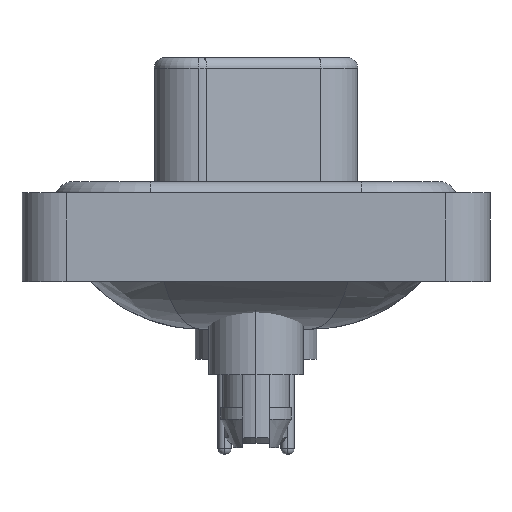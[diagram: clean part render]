
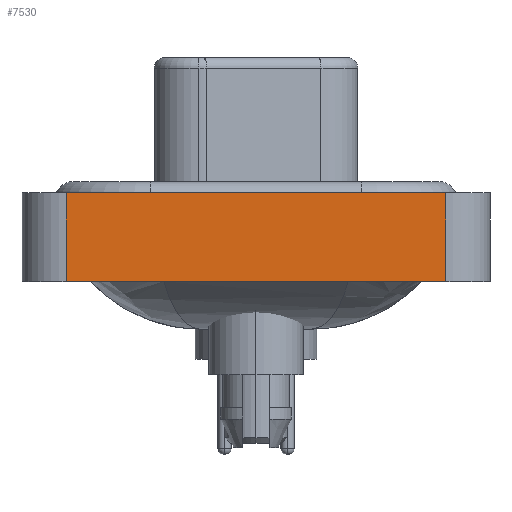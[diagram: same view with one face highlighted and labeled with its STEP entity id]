
A CAD part, left-side view. The second image highlights one B-rep face of the part: STEP entity #7530.
In plain terms, the highlighted planar face has unit normal (-1, 0, 0).
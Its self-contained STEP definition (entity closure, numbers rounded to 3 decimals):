
#92 = EDGE_CURVE ( 'NONE', #23697, #18567, #21974, .T. ) ;
#131 = VECTOR ( 'NONE', #19959, 1000. ) ;
#878 = CARTESIAN_POINT ( 'NONE',  ( -7.35, -8.55, -3.6 ) ) ;
#2245 = CARTESIAN_POINT ( 'NONE',  ( -7.35, 8.55, -3.6 ) ) ;
#3731 = ORIENTED_EDGE ( 'NONE', *, *, #8948, .F. ) ;
#3949 = ORIENTED_EDGE ( 'NONE', *, *, #6938, .T. ) ;
#5792 = LINE ( 'NONE', #7606, #18124 ) ;
#5906 = LINE ( 'NONE', #2245, #25061 ) ;
#6938 = EDGE_CURVE ( 'NONE', #8451, #23697, #22630, .T. ) ;
#7530 = ADVANCED_FACE ( 'NONE', ( #24922 ), #13343, .T. ) ;
#7606 = CARTESIAN_POINT ( 'NONE',  ( -7.35, -8.55, 0.4 ) ) ;
#8002 = CARTESIAN_POINT ( 'NONE',  ( -7.35, -8.55, -3.6 ) ) ;
#8451 = VERTEX_POINT ( 'NONE', #8697 ) ;
#8697 = CARTESIAN_POINT ( 'NONE',  ( -7.35, 8.55, -3.6 ) ) ;
#8948 = EDGE_CURVE ( 'NONE', #8451, #17237, #5906, .T. ) ;
#9150 = CARTESIAN_POINT ( 'NONE',  ( -7.35, -8.55, -3.6 ) ) ;
#9163 = EDGE_LOOP ( 'NONE', ( #20375, #23480, #3731, #3949 ) ) ;
#11244 = DIRECTION ( 'NONE',  ( -1., 0., 0. ) ) ;
#12012 = DIRECTION ( 'NONE',  ( 0., 0., 1. ) ) ;
#13085 = EDGE_CURVE ( 'NONE', #17237, #18567, #5792, .T. ) ;
#13343 = PLANE ( 'NONE',  #23044 ) ;
#14772 = CARTESIAN_POINT ( 'NONE',  ( -7.35, -8.55, 0.4 ) ) ;
#16343 = VECTOR ( 'NONE', #25719, 1000. ) ;
#17237 = VERTEX_POINT ( 'NONE', #23481 ) ;
#18124 = VECTOR ( 'NONE', #23529, 1000. ) ;
#18567 = VERTEX_POINT ( 'NONE', #14772 ) ;
#18728 = CARTESIAN_POINT ( 'NONE',  ( -7.35, -8.55, -3.6 ) ) ;
#19230 = DIRECTION ( 'NONE',  ( 0., 0., 1. ) ) ;
#19959 = DIRECTION ( 'NONE',  ( 0., -1., 0. ) ) ;
#20375 = ORIENTED_EDGE ( 'NONE', *, *, #92, .T. ) ;
#21974 = LINE ( 'NONE', #8002, #16343 ) ;
#22630 = LINE ( 'NONE', #18728, #131 ) ;
#23044 = AXIS2_PLACEMENT_3D ( 'NONE', #9150, #11244, #19230 ) ;
#23480 = ORIENTED_EDGE ( 'NONE', *, *, #13085, .F. ) ;
#23481 = CARTESIAN_POINT ( 'NONE',  ( -7.35, 8.55, 0.4 ) ) ;
#23529 = DIRECTION ( 'NONE',  ( 0., -1., 0. ) ) ;
#23697 = VERTEX_POINT ( 'NONE', #878 ) ;
#24922 = FACE_OUTER_BOUND ( 'NONE', #9163, .T. ) ;
#25061 = VECTOR ( 'NONE', #12012, 1000. ) ;
#25719 = DIRECTION ( 'NONE',  ( 0., 0., 1. ) ) ;
